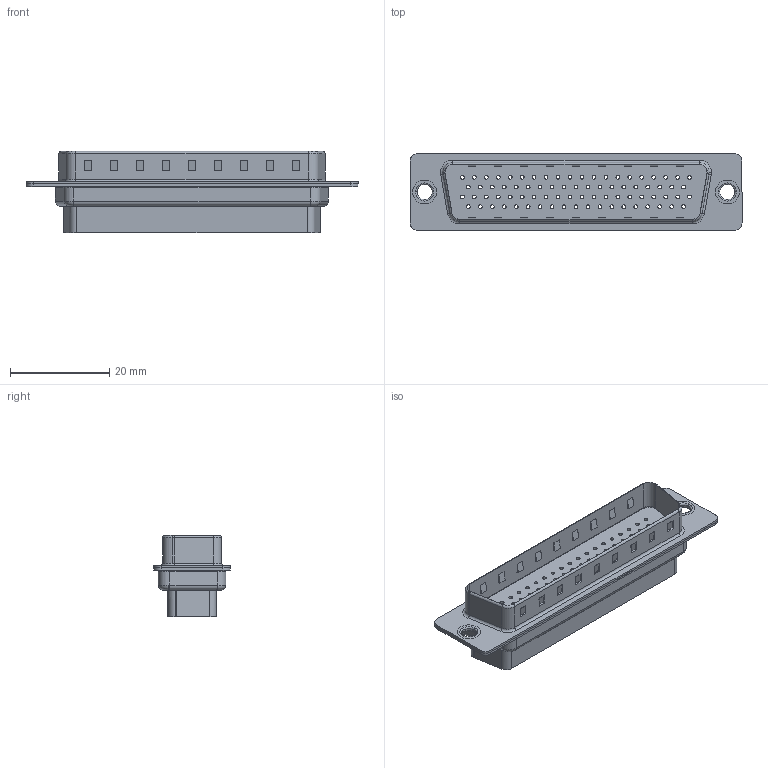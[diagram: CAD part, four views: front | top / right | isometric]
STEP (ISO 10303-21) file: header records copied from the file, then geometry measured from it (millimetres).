
FILE_DESCRIPTION (( 'STEP AP203' ), '1' );
FILE_NAME ('637-078-010-041.STEP', '2020-07-17T21:29:57', ( '' ), ( '' ), 'SwSTEP 2.0', 'SolidWorks 2020', '' );
FILE_SCHEMA (( 'CONFIG_CONTROL_DESIGN' ));
Length unit declared in the file: millimetre
Products named in the file (5): 637-078-010-041; 637 Shell Rear_78 Contacts; 637 Thru Hole Rivet; 637 Shell Front_78 Contacts; 637 Housing_78 Contacts HP
Assembly tree (5 placements, depth 2):
  637-078-010-041
    637 Housing_78 Contacts HP
    637 Shell Front_78 Contacts
    637 Shell Rear_78 Contacts
    637 Thru Hole Rivet  x2
Bounding box: 67 x 15.4 x 16.4 mm (x, y, z)
Volume: 4898.7 mm3; surface area: 10781.3 mm2
Topology: 5 solids, 5 shells, 1010 faces, 2379 edges, 1546 vertices
Faces by surface type: cylinder 593, plane 359, torus 58
Entity records: 29918 total; most frequent: DIRECTION 5557, CARTESIAN_POINT 4916, ORIENTED_EDGE 4678, EDGE_CURVE 2339, AXIS2_PLACEMENT_3D 2235, VERTEX_POINT 1522, EDGE_LOOP 1361, CIRCLE 1237
